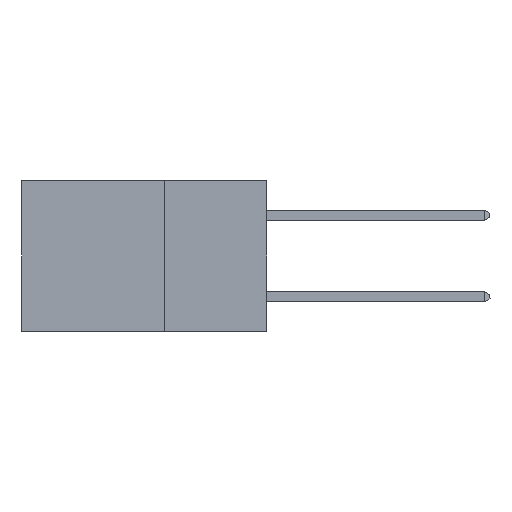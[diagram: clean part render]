
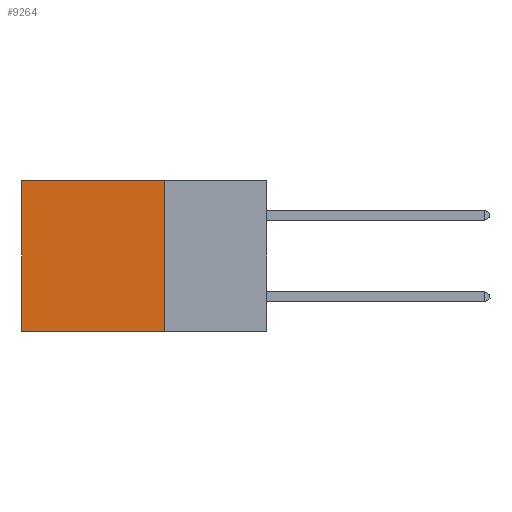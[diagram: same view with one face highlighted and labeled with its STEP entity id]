
A CAD part, left-side view. The second image highlights one B-rep face of the part: STEP entity #9264.
In plain terms, the highlighted planar face has unit normal (-1, 0, 0).
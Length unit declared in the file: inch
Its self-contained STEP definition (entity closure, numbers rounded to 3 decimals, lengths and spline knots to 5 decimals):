
#894 = DIRECTION ( 'NONE',  ( 1., 0., 0. ) ) ;
#1163 = CARTESIAN_POINT ( 'NONE',  ( 0.2875, 0.6, -0.37 ) ) ;
#1937 = DIRECTION ( 'NONE',  ( 0., 0., -1. ) ) ;
#2018 = CARTESIAN_POINT ( 'NONE',  ( 0.2875, 0.25, -0.37 ) ) ;
#3589 = CARTESIAN_POINT ( 'NONE',  ( 0.2875, 0.25, 0. ) ) ;
#3627 = DIRECTION ( 'NONE',  ( 0., 0., -1. ) ) ;
#3958 = PLANE ( 'NONE',  #14365 ) ;
#4235 = EDGE_CURVE ( 'NONE', #14631, #7450, #19351, .T. ) ;
#6082 = EDGE_CURVE ( 'NONE', #8622, #10964, #10580, .T. ) ;
#6195 = ORIENTED_EDGE ( 'NONE', *, *, #10553, .F. ) ;
#6292 = VECTOR ( 'NONE', #1937, 39.37008 ) ;
#7150 = CARTESIAN_POINT ( 'NONE',  ( 0.2875, 0.25, 0. ) ) ;
#7450 = VERTEX_POINT ( 'NONE', #1163 ) ;
#7561 = VECTOR ( 'NONE', #13172, 39.37008 ) ;
#8622 = VERTEX_POINT ( 'NONE', #12098 ) ;
#8678 = CARTESIAN_POINT ( 'NONE',  ( 0.2875, 0.25, -0.37 ) ) ;
#9264 = ADVANCED_FACE ( 'NONE', ( #18404 ), #3958, .F. ) ;
#9747 = ORIENTED_EDGE ( 'NONE', *, *, #15257, .T. ) ;
#10553 = EDGE_CURVE ( 'NONE', #10964, #7450, #11894, .T. ) ;
#10580 = LINE ( 'NONE', #13069, #6292 ) ;
#10964 = VERTEX_POINT ( 'NONE', #2018 ) ;
#11384 = VECTOR ( 'NONE', #13518, 39.37008 ) ;
#11894 = LINE ( 'NONE', #8678, #11384 ) ;
#12002 = DIRECTION ( 'NONE',  ( 0., 0., -1. ) ) ;
#12098 = CARTESIAN_POINT ( 'NONE',  ( 0.2875, 0.25, 0. ) ) ;
#13069 = CARTESIAN_POINT ( 'NONE',  ( 0.2875, 0.25, 0. ) ) ;
#13172 = DIRECTION ( 'NONE',  ( 0., 1., 0. ) ) ;
#13518 = DIRECTION ( 'NONE',  ( 0., 1., 0. ) ) ;
#14365 = AXIS2_PLACEMENT_3D ( 'NONE', #7150, #894, #12002 ) ;
#14631 = VERTEX_POINT ( 'NONE', #17695 ) ;
#14723 = ORIENTED_EDGE ( 'NONE', *, *, #4235, .T. ) ;
#14865 = ORIENTED_EDGE ( 'NONE', *, *, #6082, .F. ) ;
#15147 = VECTOR ( 'NONE', #3627, 39.37008 ) ;
#15257 = EDGE_CURVE ( 'NONE', #8622, #14631, #20293, .T. ) ;
#17695 = CARTESIAN_POINT ( 'NONE',  ( 0.2875, 0.6, 0. ) ) ;
#17912 = CARTESIAN_POINT ( 'NONE',  ( 0.2875, 0.6, 0. ) ) ;
#18404 = FACE_OUTER_BOUND ( 'NONE', #19507, .T. ) ;
#19351 = LINE ( 'NONE', #17912, #15147 ) ;
#19507 = EDGE_LOOP ( 'NONE', ( #14723, #6195, #14865, #9747 ) ) ;
#20293 = LINE ( 'NONE', #3589, #7561 ) ;
